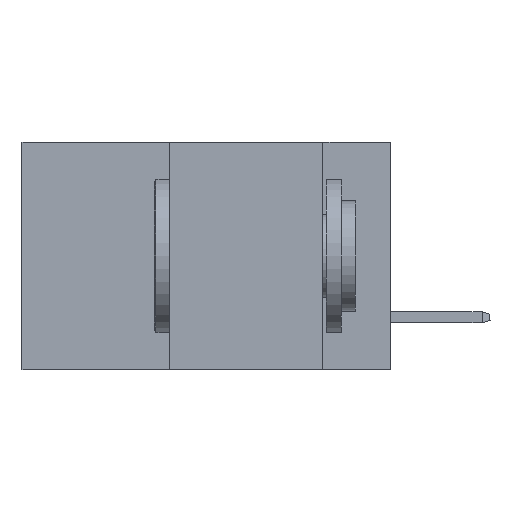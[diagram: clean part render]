
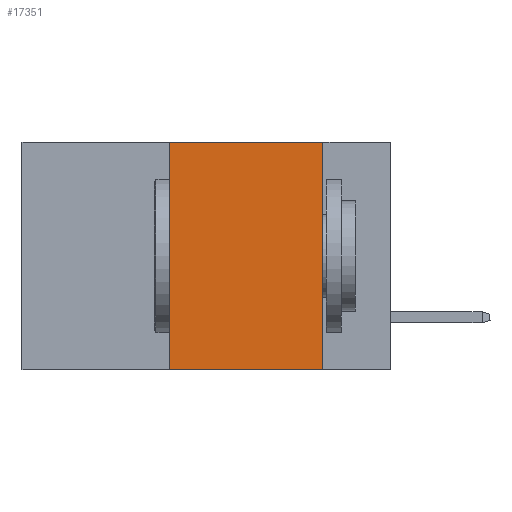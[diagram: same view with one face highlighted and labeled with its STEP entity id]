
A CAD part, left-side view. The second image highlights one B-rep face of the part: STEP entity #17351.
In plain terms, the highlighted planar face has unit normal (-1, 0, 0).
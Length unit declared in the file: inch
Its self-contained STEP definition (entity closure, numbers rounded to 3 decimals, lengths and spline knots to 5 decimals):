
#132 = VERTEX_POINT ( 'NONE', #41583 ) ;
#935 = ORIENTED_EDGE ( 'NONE', *, *, #42106, .F. ) ;
#1627 = DIRECTION ( 'NONE',  ( 0., 0., -1. ) ) ;
#1680 = ORIENTED_EDGE ( 'NONE', *, *, #8933, .T. ) ;
#1771 = DIRECTION ( 'NONE',  ( 1., 0., 0. ) ) ;
#2121 = CARTESIAN_POINT ( 'NONE',  ( 0., 0.11, -0.37 ) ) ;
#2531 = ORIENTED_EDGE ( 'NONE', *, *, #33884, .F. ) ;
#3204 = VERTEX_POINT ( 'NONE', #2121 ) ;
#3810 = LINE ( 'NONE', #10043, #15188 ) ;
#4154 = CARTESIAN_POINT ( 'NONE',  ( 0., 0.11, 0. ) ) ;
#4828 = CARTESIAN_POINT ( 'NONE',  ( 0., 0.6, 0. ) ) ;
#4896 = DIRECTION ( 'NONE',  ( 0., 0., 1. ) ) ;
#8933 = EDGE_CURVE ( 'NONE', #36441, #3204, #34987, .T. ) ;
#9954 = CARTESIAN_POINT ( 'NONE',  ( 0., 0.36, -0.37 ) ) ;
#10043 = CARTESIAN_POINT ( 'NONE',  ( 0., 0.11, 0. ) ) ;
#11815 = LINE ( 'NONE', #33255, #22167 ) ;
#13359 = DIRECTION ( 'NONE',  ( 0., -1., 0. ) ) ;
#14773 = PLANE ( 'NONE',  #34380 ) ;
#15188 = VECTOR ( 'NONE', #16957, 39.37008 ) ;
#16957 = DIRECTION ( 'NONE',  ( 0., 0., -1. ) ) ;
#17351 = ADVANCED_FACE ( 'NONE', ( #40687 ), #14773, .F. ) ;
#17655 = EDGE_CURVE ( 'NONE', #20169, #3204, #3810, .T. ) ;
#18050 = CARTESIAN_POINT ( 'NONE',  ( 0., 0.36, 0. ) ) ;
#20169 = VERTEX_POINT ( 'NONE', #4154 ) ;
#22167 = VECTOR ( 'NONE', #13359, 39.37008 ) ;
#29454 = CARTESIAN_POINT ( 'NONE',  ( 0., 0.6, -0.37 ) ) ;
#33255 = CARTESIAN_POINT ( 'NONE',  ( 0., 0.6, 0. ) ) ;
#33884 = EDGE_CURVE ( 'NONE', #132, #20169, #11815, .T. ) ;
#34380 = AXIS2_PLACEMENT_3D ( 'NONE', #4828, #1771, #1627 ) ;
#34987 = LINE ( 'NONE', #29454, #42786 ) ;
#35100 = ORIENTED_EDGE ( 'NONE', *, *, #17655, .F. ) ;
#36441 = VERTEX_POINT ( 'NONE', #9954 ) ;
#37279 = LINE ( 'NONE', #18050, #38868 ) ;
#38868 = VECTOR ( 'NONE', #4896, 39.37008 ) ;
#39615 = DIRECTION ( 'NONE',  ( 0., -1., 0. ) ) ;
#40687 = FACE_OUTER_BOUND ( 'NONE', #42743, .T. ) ;
#41583 = CARTESIAN_POINT ( 'NONE',  ( 0., 0.36, 0. ) ) ;
#42106 = EDGE_CURVE ( 'NONE', #36441, #132, #37279, .T. ) ;
#42743 = EDGE_LOOP ( 'NONE', ( #35100, #2531, #935, #1680 ) ) ;
#42786 = VECTOR ( 'NONE', #39615, 39.37008 ) ;
